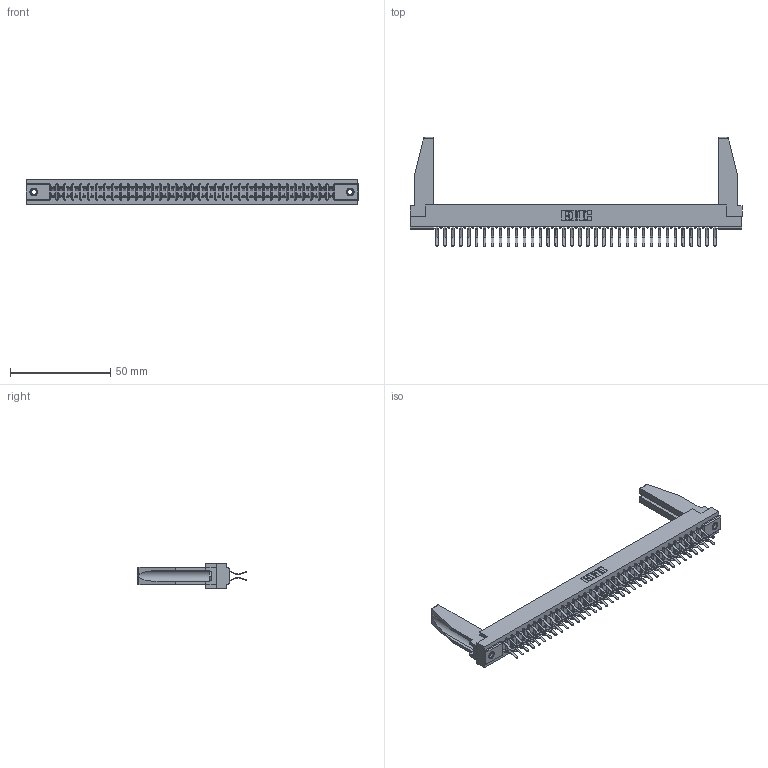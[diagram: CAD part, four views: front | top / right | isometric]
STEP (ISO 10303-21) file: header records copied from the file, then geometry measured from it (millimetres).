
FILE_DESCRIPTION (( 'STEP AP203' ), '1' );
FILE_NAME ('307-072-460-278.STEP', '2020-10-01T02:45:55', ( '' ), ( '' ), 'SwSTEP 2.0', 'SolidWorks 2020', '' );
FILE_SCHEMA (( 'CONFIG_CONTROL_DESIGN' ));
Length unit declared in the file: inch
Products named in the file (5): 345-250-001_345-250-001-102; 307-072-460-278; 307-220-078; 307 Part_.156 Dia Mounting Holes; 307-290-001_560
Assembly tree (77 placements, depth 2):
  307-072-460-278
    307 Part_.156 Dia Mounting Holes
    307-290-001_560  x72
    307-220-078  x2
    345-250-001_345-250-001-102  x2
Bounding box: 165.66 x 54.43 x 12.7 mm (x, y, z)
Volume: 21656.4 mm3; surface area: 25800.4 mm2
Topology: 77 solids, 77 shells, 3885 faces, 10877 edges, 7046 vertices
Faces by surface type: plane 2530, cylinder 1265, sphere 74, cone 12, torus 4
Entity records: 35297 total; most frequent: CARTESIAN_POINT 5786, ORIENTED_EDGE 5692, DIRECTION 5624, EDGE_CURVE 2846, LINE 2184, VECTOR 2184, VERTEX_POINT 1840, AXIS2_PLACEMENT_3D 1720
